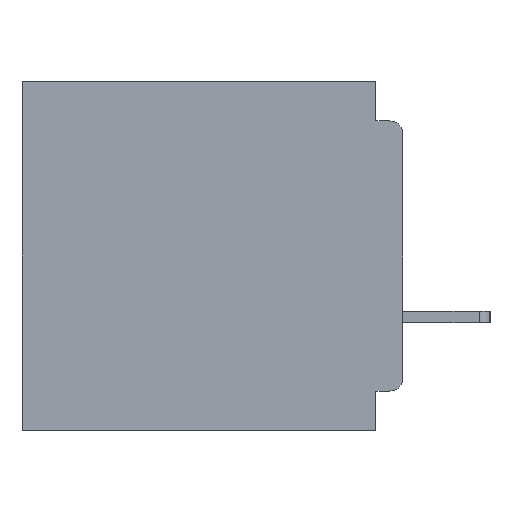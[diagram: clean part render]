
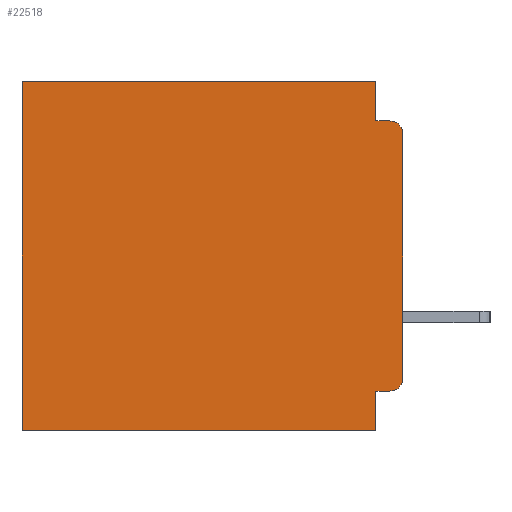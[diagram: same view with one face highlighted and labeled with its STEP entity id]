
A CAD part, left-side view. The second image highlights one B-rep face of the part: STEP entity #22518.
In plain terms, the highlighted planar face has unit normal (-1, 0, 0).
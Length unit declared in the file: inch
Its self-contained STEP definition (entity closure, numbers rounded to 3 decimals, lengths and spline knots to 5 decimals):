
#502 = VERTEX_POINT ( 'NONE', #32369 ) ;
#1075 = CARTESIAN_POINT ( 'NONE',  ( 0.3, 0., -0.045 ) ) ;
#1264 = LINE ( 'NONE', #35559, #26074 ) ;
#1357 = ORIENTED_EDGE ( 'NONE', *, *, #15567, .F. ) ;
#1362 = VERTEX_POINT ( 'NONE', #38722 ) ;
#1647 = EDGE_CURVE ( 'NONE', #12390, #12897, #15382, .T. ) ;
#2464 = CARTESIAN_POINT ( 'NONE',  ( 0.3, 0.031, -0.4 ) ) ;
#2533 = ORIENTED_EDGE ( 'NONE', *, *, #3338, .F. ) ;
#2741 = DIRECTION ( 'NONE',  ( 0., 0., -1. ) ) ;
#3338 = EDGE_CURVE ( 'NONE', #5609, #10776, #23746, .T. ) ;
#3579 = VECTOR ( 'NONE', #16136, 39.37008 ) ;
#3642 = LINE ( 'NONE', #5418, #30423 ) ;
#4482 = CARTESIAN_POINT ( 'NONE',  ( 0.3, 0., -0.4 ) ) ;
#5418 = CARTESIAN_POINT ( 'NONE',  ( 0.3, 0., -0.4 ) ) ;
#5436 = CARTESIAN_POINT ( 'NONE',  ( 0.3, 0.437, 0. ) ) ;
#5609 = VERTEX_POINT ( 'NONE', #18491 ) ;
#5621 = CARTESIAN_POINT ( 'NONE',  ( 0.3, 0.015, -0.06 ) ) ;
#5832 = DIRECTION ( 'NONE',  ( -1., 0., 0. ) ) ;
#6160 = EDGE_CURVE ( 'NONE', #1362, #5609, #23509, .T. ) ;
#6217 = LINE ( 'NONE', #4482, #37456 ) ;
#6320 = CARTESIAN_POINT ( 'NONE',  ( 0.3, 0., -0.06 ) ) ;
#7004 = ORIENTED_EDGE ( 'NONE', *, *, #1647, .T. ) ;
#7046 = ORIENTED_EDGE ( 'NONE', *, *, #32478, .F. ) ;
#8358 = VERTEX_POINT ( 'NONE', #41197 ) ;
#10352 = EDGE_CURVE ( 'NONE', #35378, #30652, #1264, .T. ) ;
#10504 = AXIS2_PLACEMENT_3D ( 'NONE', #18920, #22138, #2741 ) ;
#10770 = DIRECTION ( 'NONE',  ( 0., 1., 0. ) ) ;
#10776 = VERTEX_POINT ( 'NONE', #18955 ) ;
#11542 = FACE_OUTER_BOUND ( 'NONE', #15923, .T. ) ;
#12390 = VERTEX_POINT ( 'NONE', #6320 ) ;
#12827 = ORIENTED_EDGE ( 'NONE', *, *, #34331, .T. ) ;
#12897 = VERTEX_POINT ( 'NONE', #34596 ) ;
#13527 = AXIS2_PLACEMENT_3D ( 'NONE', #35694, #16479, #38936 ) ;
#14242 = VECTOR ( 'NONE', #28316, 39.37008 ) ;
#15382 = CIRCLE ( 'NONE', #27722, 0.015 ) ;
#15567 = EDGE_CURVE ( 'NONE', #8358, #12897, #16156, .T. ) ;
#15722 = PLANE ( 'NONE',  #10504 ) ;
#15923 = EDGE_LOOP ( 'NONE', ( #38705, #7004, #1357, #7046, #30234, #26775, #32832, #2533, #25830, #12827 ) ) ;
#16136 = DIRECTION ( 'NONE',  ( 0., 0., -1. ) ) ;
#16156 = LINE ( 'NONE', #1075, #40754 ) ;
#16333 = DIRECTION ( 'NONE',  ( 0., 0., -1. ) ) ;
#16460 = VERTEX_POINT ( 'NONE', #28991 ) ;
#16479 = DIRECTION ( 'NONE',  ( -1., 0., 0. ) ) ;
#16663 = CIRCLE ( 'NONE', #13527, 0.015 ) ;
#17293 = CARTESIAN_POINT ( 'NONE',  ( 0.3, 0.437, -0.4 ) ) ;
#17904 = DIRECTION ( 'NONE',  ( 0., 0., -1. ) ) ;
#18036 = CARTESIAN_POINT ( 'NONE',  ( 0.3, 0., -0.355 ) ) ;
#18491 = CARTESIAN_POINT ( 'NONE',  ( 0.3, 0.031, -0.355 ) ) ;
#18805 = EDGE_CURVE ( 'NONE', #10776, #30652, #6217, .T. ) ;
#18920 = CARTESIAN_POINT ( 'NONE',  ( 0.3, 0., -0.4 ) ) ;
#18955 = CARTESIAN_POINT ( 'NONE',  ( 0.3, 0.031, -0.4 ) ) ;
#19276 = EDGE_CURVE ( 'NONE', #16460, #35378, #19341, .T. ) ;
#19341 = LINE ( 'NONE', #26782, #20346 ) ;
#20346 = VECTOR ( 'NONE', #10770, 39.37008 ) ;
#20515 = DIRECTION ( 'NONE',  ( 0., -1., 0. ) ) ;
#20807 = LINE ( 'NONE', #32106, #3579 ) ;
#22138 = DIRECTION ( 'NONE',  ( 1., 0., 0. ) ) ;
#22518 = ADVANCED_FACE ( 'NONE', ( #11542 ), #15722, .F. ) ;
#23509 = LINE ( 'NONE', #18036, #32052 ) ;
#23746 = LINE ( 'NONE', #2464, #14242 ) ;
#24337 = DIRECTION ( 'NONE',  ( 0., 1., 0. ) ) ;
#24770 = DIRECTION ( 'NONE',  ( 0., 0., -1. ) ) ;
#25830 = ORIENTED_EDGE ( 'NONE', *, *, #6160, .F. ) ;
#26074 = VECTOR ( 'NONE', #16333, 39.37008 ) ;
#26775 = ORIENTED_EDGE ( 'NONE', *, *, #10352, .T. ) ;
#26782 = CARTESIAN_POINT ( 'NONE',  ( 0.3, 0., 0. ) ) ;
#27190 = EDGE_CURVE ( 'NONE', #12390, #502, #3642, .T. ) ;
#27722 = AXIS2_PLACEMENT_3D ( 'NONE', #5621, #5832, #17904 ) ;
#28316 = DIRECTION ( 'NONE',  ( 0., 0., -1. ) ) ;
#28991 = CARTESIAN_POINT ( 'NONE',  ( 0.3, 0.031, 0. ) ) ;
#30234 = ORIENTED_EDGE ( 'NONE', *, *, #19276, .T. ) ;
#30315 = DIRECTION ( 'NONE',  ( 0., 1., 0. ) ) ;
#30423 = VECTOR ( 'NONE', #24770, 39.37008 ) ;
#30652 = VERTEX_POINT ( 'NONE', #17293 ) ;
#32052 = VECTOR ( 'NONE', #24337, 39.37008 ) ;
#32106 = CARTESIAN_POINT ( 'NONE',  ( 0.3, 0.031, 0. ) ) ;
#32369 = CARTESIAN_POINT ( 'NONE',  ( 0.3, 0., -0.34 ) ) ;
#32478 = EDGE_CURVE ( 'NONE', #16460, #8358, #20807, .T. ) ;
#32832 = ORIENTED_EDGE ( 'NONE', *, *, #18805, .F. ) ;
#34331 = EDGE_CURVE ( 'NONE', #1362, #502, #16663, .T. ) ;
#34596 = CARTESIAN_POINT ( 'NONE',  ( 0.3, 0.015, -0.045 ) ) ;
#35378 = VERTEX_POINT ( 'NONE', #5436 ) ;
#35559 = CARTESIAN_POINT ( 'NONE',  ( 0.3, 0.437, -0.4 ) ) ;
#35694 = CARTESIAN_POINT ( 'NONE',  ( 0.3, 0.015, -0.34 ) ) ;
#37456 = VECTOR ( 'NONE', #30315, 39.37008 ) ;
#38705 = ORIENTED_EDGE ( 'NONE', *, *, #27190, .F. ) ;
#38722 = CARTESIAN_POINT ( 'NONE',  ( 0.3, 0.015, -0.355 ) ) ;
#38936 = DIRECTION ( 'NONE',  ( 0., 0., -1. ) ) ;
#40754 = VECTOR ( 'NONE', #20515, 39.37008 ) ;
#41197 = CARTESIAN_POINT ( 'NONE',  ( 0.3, 0.031, -0.045 ) ) ;
